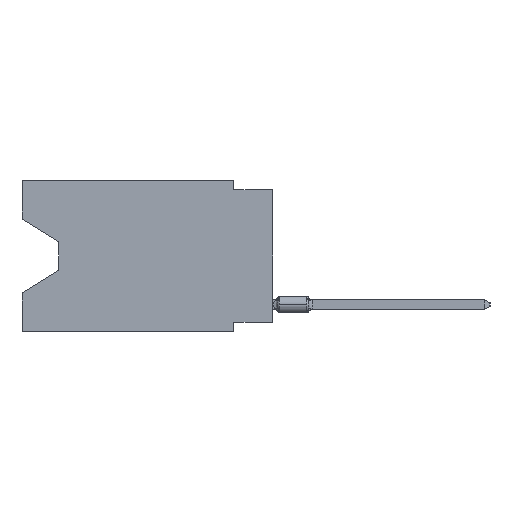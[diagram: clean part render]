
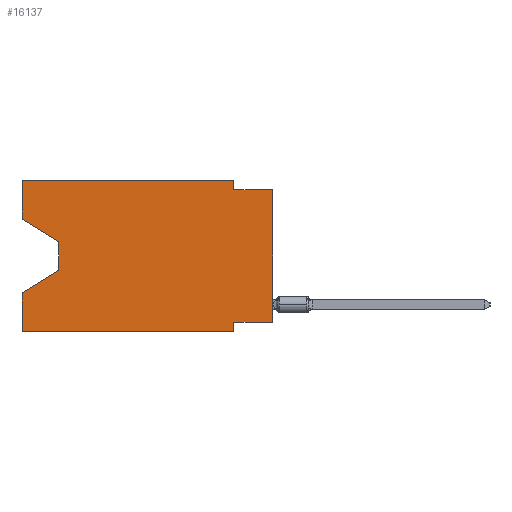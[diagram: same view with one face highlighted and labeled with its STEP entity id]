
A CAD part, left-side view. The second image highlights one B-rep face of the part: STEP entity #16137.
In plain terms, the highlighted planar face has unit normal (-1, 0, 0).
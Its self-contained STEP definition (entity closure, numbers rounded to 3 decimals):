
#213 = ORIENTED_EDGE ( 'NONE', *, *, #14254, .T. ) ;
#510 = CARTESIAN_POINT ( 'NONE',  ( 0., 16.383, -9.906 ) ) ;
#966 = ORIENTED_EDGE ( 'NONE', *, *, #3225, .F. ) ;
#1247 = LINE ( 'NONE', #10250, #8505 ) ;
#1425 = LINE ( 'NONE', #6282, #28991 ) ;
#2185 = LINE ( 'NONE', #15189, #20131 ) ;
#2768 = ORIENTED_EDGE ( 'NONE', *, *, #8130, .F. ) ;
#3083 = VECTOR ( 'NONE', #26644, 1000. ) ;
#3225 = EDGE_CURVE ( 'NONE', #16012, #16536, #16480, .T. ) ;
#3513 = VERTEX_POINT ( 'NONE', #25315 ) ;
#3790 = VERTEX_POINT ( 'NONE', #25277 ) ;
#4035 = ORIENTED_EDGE ( 'NONE', *, *, #12891, .F. ) ;
#4424 = VERTEX_POINT ( 'NONE', #17241 ) ;
#5794 = DIRECTION ( 'NONE',  ( 0., 0., -1. ) ) ;
#6129 = VECTOR ( 'NONE', #24471, 1000. ) ;
#6282 = CARTESIAN_POINT ( 'NONE',  ( 0., 13.97, -4.013 ) ) ;
#6582 = EDGE_CURVE ( 'NONE', #7125, #22549, #22062, .T. ) ;
#6877 = VECTOR ( 'NONE', #25072, 1000. ) ;
#7125 = VERTEX_POINT ( 'NONE', #13716 ) ;
#7179 = EDGE_CURVE ( 'NONE', #3513, #3790, #7504, .T. ) ;
#7355 = CARTESIAN_POINT ( 'NONE',  ( 0., 16.383, 0. ) ) ;
#7487 = VERTEX_POINT ( 'NONE', #24415 ) ;
#7504 = LINE ( 'NONE', #23061, #8416 ) ;
#7642 = LINE ( 'NONE', #14304, #23285 ) ;
#7704 = EDGE_CURVE ( 'NONE', #17720, #15601, #13084, .T. ) ;
#8130 = EDGE_CURVE ( 'NONE', #4424, #15601, #20181, .T. ) ;
#8267 = ORIENTED_EDGE ( 'NONE', *, *, #7704, .T. ) ;
#8416 = VECTOR ( 'NONE', #14311, 1000. ) ;
#8505 = VECTOR ( 'NONE', #17475, 1000. ) ;
#8510 = CARTESIAN_POINT ( 'NONE',  ( 0., 0., 0. ) ) ;
#8833 = CARTESIAN_POINT ( 'NONE',  ( 0., 13.97, -4.013 ) ) ;
#9371 = VERTEX_POINT ( 'NONE', #22656 ) ;
#9398 = ORIENTED_EDGE ( 'NONE', *, *, #20574, .F. ) ;
#9762 = AXIS2_PLACEMENT_3D ( 'NONE', #12876, #26366, #5794 ) ;
#10250 = CARTESIAN_POINT ( 'NONE',  ( 0., 16.383, 0. ) ) ;
#10500 = ORIENTED_EDGE ( 'NONE', *, *, #10536, .F. ) ;
#10536 = EDGE_CURVE ( 'NONE', #17720, #3790, #1247, .T. ) ;
#10842 = CARTESIAN_POINT ( 'NONE',  ( 0., 2.54, -9.906 ) ) ;
#11613 = LINE ( 'NONE', #25382, #6877 ) ;
#12363 = DIRECTION ( 'NONE',  ( 0., -1., 0. ) ) ;
#12876 = CARTESIAN_POINT ( 'NONE',  ( 0., 16.383, 0. ) ) ;
#12891 = EDGE_CURVE ( 'NONE', #17178, #9371, #7642, .T. ) ;
#13084 = LINE ( 'NONE', #24617, #14594 ) ;
#13716 = CARTESIAN_POINT ( 'NONE',  ( 0., 16.383, -2.546 ) ) ;
#14254 = EDGE_CURVE ( 'NONE', #22549, #3513, #1425, .T. ) ;
#14304 = CARTESIAN_POINT ( 'NONE',  ( 0., 16.383, 0. ) ) ;
#14311 = DIRECTION ( 'NONE',  ( 0., 0.855, -0.519 ) ) ;
#14594 = VECTOR ( 'NONE', #19622, 1000. ) ;
#14819 = FACE_OUTER_BOUND ( 'NONE', #22014, .T. ) ;
#15189 = CARTESIAN_POINT ( 'NONE',  ( 0., 2.54, 0. ) ) ;
#15601 = VERTEX_POINT ( 'NONE', #18422 ) ;
#15781 = DIRECTION ( 'NONE',  ( 0., 0., -1. ) ) ;
#16012 = VERTEX_POINT ( 'NONE', #25350 ) ;
#16062 = ORIENTED_EDGE ( 'NONE', *, *, #7179, .T. ) ;
#16137 = ADVANCED_FACE ( 'NONE', ( #14819 ), #17027, .F. ) ;
#16480 = LINE ( 'NONE', #21229, #22478 ) ;
#16536 = VERTEX_POINT ( 'NONE', #25895 ) ;
#16630 = ORIENTED_EDGE ( 'NONE', *, *, #22007, .F. ) ;
#17027 = PLANE ( 'NONE',  #9762 ) ;
#17178 = VERTEX_POINT ( 'NONE', #7355 ) ;
#17241 = CARTESIAN_POINT ( 'NONE',  ( 0., 2.54, -9.271 ) ) ;
#17410 = LINE ( 'NONE', #8510, #22782 ) ;
#17459 = LINE ( 'NONE', #26487, #3083 ) ;
#17465 = ORIENTED_EDGE ( 'NONE', *, *, #21239, .F. ) ;
#17475 = DIRECTION ( 'NONE',  ( 0., 0., 1. ) ) ;
#17720 = VERTEX_POINT ( 'NONE', #510 ) ;
#18422 = CARTESIAN_POINT ( 'NONE',  ( 0., 2.54, -9.906 ) ) ;
#19023 = DIRECTION ( 'NONE',  ( 0., -1., 0. ) ) ;
#19622 = DIRECTION ( 'NONE',  ( 0., -1., 0. ) ) ;
#19769 = ORIENTED_EDGE ( 'NONE', *, *, #28549, .T. ) ;
#19831 = CARTESIAN_POINT ( 'NONE',  ( 0., 16.383, -2.546 ) ) ;
#20131 = VECTOR ( 'NONE', #15781, 1000. ) ;
#20181 = LINE ( 'NONE', #10842, #6129 ) ;
#20574 = EDGE_CURVE ( 'NONE', #7487, #4424, #11613, .T. ) ;
#21229 = CARTESIAN_POINT ( 'NONE',  ( 0., 0., -0.635 ) ) ;
#21239 = EDGE_CURVE ( 'NONE', #9371, #16012, #2185, .T. ) ;
#21486 = ORIENTED_EDGE ( 'NONE', *, *, #6582, .T. ) ;
#21577 = DIRECTION ( 'NONE',  ( 0., 0., 1. ) ) ;
#22007 = EDGE_CURVE ( 'NONE', #7125, #17178, #17459, .T. ) ;
#22014 = EDGE_LOOP ( 'NONE', ( #21486, #213, #16062, #10500, #8267, #2768, #9398, #19769, #966, #17465, #4035, #16630 ) ) ;
#22062 = LINE ( 'NONE', #19831, #24451 ) ;
#22478 = VECTOR ( 'NONE', #19023, 1000. ) ;
#22549 = VERTEX_POINT ( 'NONE', #8833 ) ;
#22656 = CARTESIAN_POINT ( 'NONE',  ( 0., 2.54, 0. ) ) ;
#22782 = VECTOR ( 'NONE', #21577, 1000. ) ;
#23061 = CARTESIAN_POINT ( 'NONE',  ( 0., 13.97, -5.893 ) ) ;
#23285 = VECTOR ( 'NONE', #12363, 1000. ) ;
#24415 = CARTESIAN_POINT ( 'NONE',  ( 0., 0., -9.271 ) ) ;
#24451 = VECTOR ( 'NONE', #26795, 1000. ) ;
#24471 = DIRECTION ( 'NONE',  ( 0., 0., -1. ) ) ;
#24617 = CARTESIAN_POINT ( 'NONE',  ( 0., 16.383, -9.906 ) ) ;
#25072 = DIRECTION ( 'NONE',  ( 0., 1., 0. ) ) ;
#25277 = CARTESIAN_POINT ( 'NONE',  ( 0., 16.383, -7.36 ) ) ;
#25315 = CARTESIAN_POINT ( 'NONE',  ( 0., 13.97, -5.893 ) ) ;
#25350 = CARTESIAN_POINT ( 'NONE',  ( 0., 2.54, -0.635 ) ) ;
#25382 = CARTESIAN_POINT ( 'NONE',  ( 0., 0., -9.271 ) ) ;
#25895 = CARTESIAN_POINT ( 'NONE',  ( 0., 0., -0.635 ) ) ;
#26366 = DIRECTION ( 'NONE',  ( 1., 0., 0. ) ) ;
#26487 = CARTESIAN_POINT ( 'NONE',  ( 0., 16.383, 0. ) ) ;
#26644 = DIRECTION ( 'NONE',  ( 0., 0., 1. ) ) ;
#26710 = DIRECTION ( 'NONE',  ( 0., 0., -1. ) ) ;
#26795 = DIRECTION ( 'NONE',  ( 0., -0.855, -0.519 ) ) ;
#28549 = EDGE_CURVE ( 'NONE', #7487, #16536, #17410, .T. ) ;
#28991 = VECTOR ( 'NONE', #26710, 1000. ) ;
